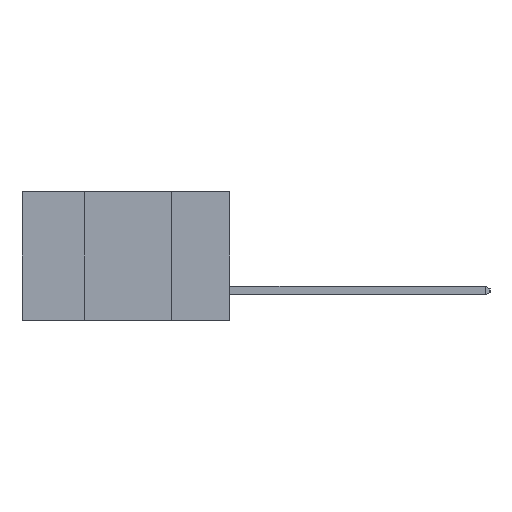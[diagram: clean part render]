
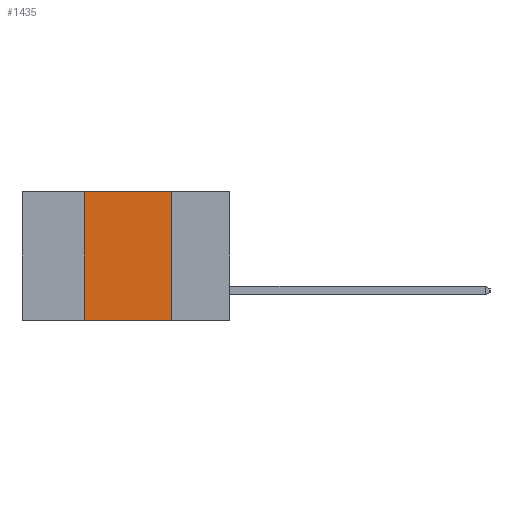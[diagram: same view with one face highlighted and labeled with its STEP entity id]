
A CAD part, left-side view. The second image highlights one B-rep face of the part: STEP entity #1435.
In plain terms, the highlighted planar face has unit normal (-1, 0, 0).
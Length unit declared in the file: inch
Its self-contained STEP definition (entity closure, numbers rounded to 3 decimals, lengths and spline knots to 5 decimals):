
#1170 = CARTESIAN_POINT ( 'NONE',  ( 0., 0.42, -0.37 ) ) ;
#1435 = ADVANCED_FACE ( 'NONE', ( #10543 ), #13240, .F. ) ;
#2302 = VECTOR ( 'NONE', #8937, 39.37008 ) ;
#3883 = VECTOR ( 'NONE', #15000, 39.37008 ) ;
#4270 = ORIENTED_EDGE ( 'NONE', *, *, #15387, .F. ) ;
#4555 = VERTEX_POINT ( 'NONE', #14499 ) ;
#5654 = EDGE_LOOP ( 'NONE', ( #4270, #11528, #18489, #18067 ) ) ;
#6013 = LINE ( 'NONE', #7513, #17433 ) ;
#6260 = LINE ( 'NONE', #16052, #2302 ) ;
#6556 = VECTOR ( 'NONE', #16137, 39.37008 ) ;
#7031 = DIRECTION ( 'NONE',  ( 1., 0., 0. ) ) ;
#7513 = CARTESIAN_POINT ( 'NONE',  ( 0., 0.17, -0.37 ) ) ;
#7857 = CARTESIAN_POINT ( 'NONE',  ( 0., 0.42, -0.37 ) ) ;
#8937 = DIRECTION ( 'NONE',  ( 0., -1., 0. ) ) ;
#8946 = DIRECTION ( 'NONE',  ( 0., 0., -1. ) ) ;
#9033 = CARTESIAN_POINT ( 'NONE',  ( 0., 0.6, -0.37 ) ) ;
#10168 = CARTESIAN_POINT ( 'NONE',  ( 0., 0.17, 0. ) ) ;
#10543 = FACE_OUTER_BOUND ( 'NONE', #5654, .T. ) ;
#11528 = ORIENTED_EDGE ( 'NONE', *, *, #14674, .F. ) ;
#11874 = EDGE_CURVE ( 'NONE', #15261, #4555, #12073, .T. ) ;
#12073 = LINE ( 'NONE', #7857, #3883 ) ;
#12084 = CARTESIAN_POINT ( 'NONE',  ( 0., 0.6, 0. ) ) ;
#12913 = VERTEX_POINT ( 'NONE', #15646 ) ;
#13163 = EDGE_CURVE ( 'NONE', #15261, #12913, #17925, .T. ) ;
#13240 = PLANE ( 'NONE',  #15461 ) ;
#14499 = CARTESIAN_POINT ( 'NONE',  ( 0., 0.42, 0. ) ) ;
#14674 = EDGE_CURVE ( 'NONE', #4555, #18347, #6260, .T. ) ;
#15000 = DIRECTION ( 'NONE',  ( 0., 0., 1. ) ) ;
#15261 = VERTEX_POINT ( 'NONE', #1170 ) ;
#15387 = EDGE_CURVE ( 'NONE', #18347, #12913, #6013, .T. ) ;
#15461 = AXIS2_PLACEMENT_3D ( 'NONE', #12084, #7031, #8946 ) ;
#15646 = CARTESIAN_POINT ( 'NONE',  ( 0., 0.17, -0.37 ) ) ;
#16052 = CARTESIAN_POINT ( 'NONE',  ( 0., 0.6, 0. ) ) ;
#16137 = DIRECTION ( 'NONE',  ( 0., -1., 0. ) ) ;
#17433 = VECTOR ( 'NONE', #17491, 39.37008 ) ;
#17491 = DIRECTION ( 'NONE',  ( 0., 0., -1. ) ) ;
#17925 = LINE ( 'NONE', #9033, #6556 ) ;
#18067 = ORIENTED_EDGE ( 'NONE', *, *, #13163, .T. ) ;
#18347 = VERTEX_POINT ( 'NONE', #10168 ) ;
#18489 = ORIENTED_EDGE ( 'NONE', *, *, #11874, .F. ) ;
